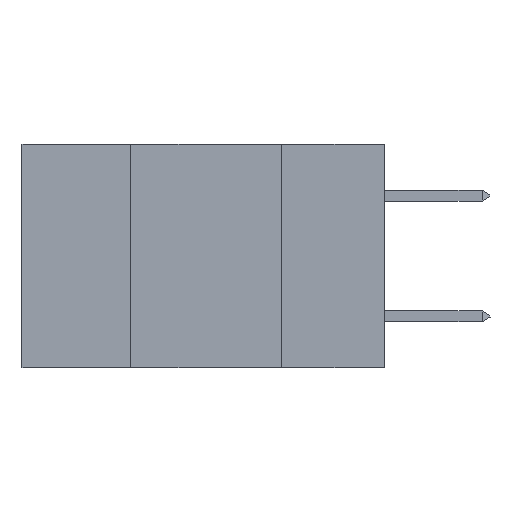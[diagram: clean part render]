
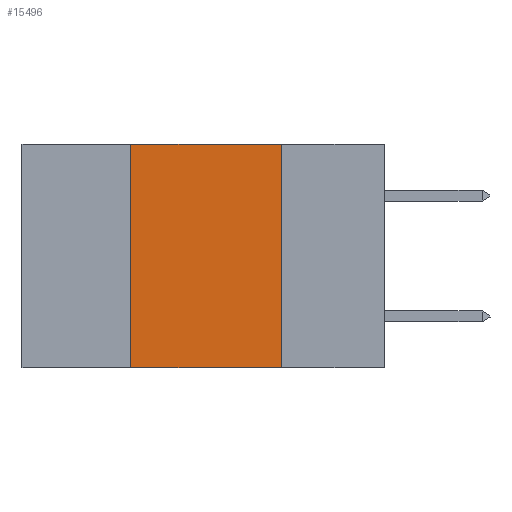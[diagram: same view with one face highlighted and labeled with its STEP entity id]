
A CAD part, left-side view. The second image highlights one B-rep face of the part: STEP entity #15496.
In plain terms, the highlighted planar face has unit normal (-1, 0, 0).
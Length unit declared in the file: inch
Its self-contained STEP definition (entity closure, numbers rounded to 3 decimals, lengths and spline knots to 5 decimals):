
#232 = CARTESIAN_POINT ( 'NONE',  ( 0., 0.6, 0. ) ) ;
#262 = VERTEX_POINT ( 'NONE', #6751 ) ;
#1526 = CARTESIAN_POINT ( 'NONE',  ( 0., 0.6, 0. ) ) ;
#2187 = CARTESIAN_POINT ( 'NONE',  ( 0., 0.17, 0. ) ) ;
#2855 = DIRECTION ( 'NONE',  ( 0., 0., -1. ) ) ;
#3026 = CARTESIAN_POINT ( 'NONE',  ( 0., 0.42, 0. ) ) ;
#3160 = LINE ( 'NONE', #13408, #4375 ) ;
#3994 = ORIENTED_EDGE ( 'NONE', *, *, #4071, .F. ) ;
#4071 = EDGE_CURVE ( 'NONE', #16138, #7040, #12730, .T. ) ;
#4194 = AXIS2_PLACEMENT_3D ( 'NONE', #1526, #11814, #2855 ) ;
#4375 = VECTOR ( 'NONE', #5616, 39.37008 ) ;
#4791 = LINE ( 'NONE', #3026, #14762 ) ;
#5276 = CARTESIAN_POINT ( 'NONE',  ( 0., 0.42, -0.37 ) ) ;
#5309 = DIRECTION ( 'NONE',  ( 0., 0., -1. ) ) ;
#5616 = DIRECTION ( 'NONE',  ( 0., -1., 0. ) ) ;
#6456 = EDGE_LOOP ( 'NONE', ( #9789, #3994, #15592, #10648 ) ) ;
#6751 = CARTESIAN_POINT ( 'NONE',  ( 0., 0.17, -0.37 ) ) ;
#6813 = LINE ( 'NONE', #2187, #14138 ) ;
#7040 = VERTEX_POINT ( 'NONE', #10731 ) ;
#8125 = FACE_OUTER_BOUND ( 'NONE', #6456, .T. ) ;
#8227 = DIRECTION ( 'NONE',  ( 0., 0., 1. ) ) ;
#8829 = EDGE_CURVE ( 'NONE', #10185, #16138, #4791, .T. ) ;
#9789 = ORIENTED_EDGE ( 'NONE', *, *, #12581, .F. ) ;
#10185 = VERTEX_POINT ( 'NONE', #5276 ) ;
#10648 = ORIENTED_EDGE ( 'NONE', *, *, #12868, .T. ) ;
#10684 = PLANE ( 'NONE',  #4194 ) ;
#10731 = CARTESIAN_POINT ( 'NONE',  ( 0., 0.17, 0. ) ) ;
#11420 = CARTESIAN_POINT ( 'NONE',  ( 0., 0.42, 0. ) ) ;
#11706 = VECTOR ( 'NONE', #15652, 39.37008 ) ;
#11814 = DIRECTION ( 'NONE',  ( 1., 0., 0. ) ) ;
#12581 = EDGE_CURVE ( 'NONE', #7040, #262, #6813, .T. ) ;
#12730 = LINE ( 'NONE', #232, #11706 ) ;
#12868 = EDGE_CURVE ( 'NONE', #10185, #262, #3160, .T. ) ;
#13408 = CARTESIAN_POINT ( 'NONE',  ( 0., 0.6, -0.37 ) ) ;
#14138 = VECTOR ( 'NONE', #5309, 39.37008 ) ;
#14762 = VECTOR ( 'NONE', #8227, 39.37008 ) ;
#15496 = ADVANCED_FACE ( 'NONE', ( #8125 ), #10684, .F. ) ;
#15592 = ORIENTED_EDGE ( 'NONE', *, *, #8829, .F. ) ;
#15652 = DIRECTION ( 'NONE',  ( 0., -1., 0. ) ) ;
#16138 = VERTEX_POINT ( 'NONE', #11420 ) ;
